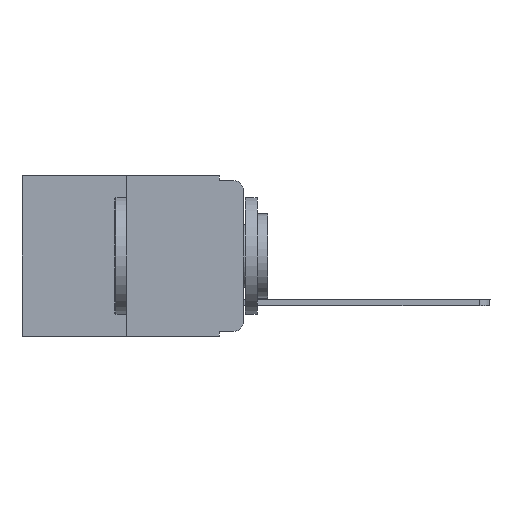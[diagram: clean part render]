
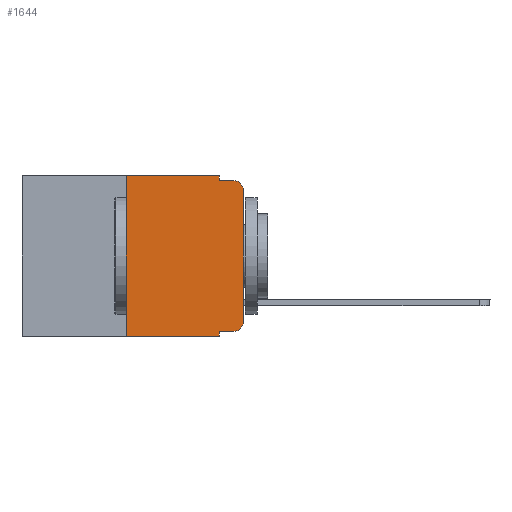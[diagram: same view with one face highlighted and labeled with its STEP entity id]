
A CAD part, left-side view. The second image highlights one B-rep face of the part: STEP entity #1644.
In plain terms, the highlighted planar face has unit normal (-1, 0, 0).
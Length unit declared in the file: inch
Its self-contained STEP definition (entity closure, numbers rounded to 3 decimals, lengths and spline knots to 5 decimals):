
#86 = EDGE_CURVE ( 'NONE', #6465, #8128, #5907, .T. ) ;
#367 = EDGE_CURVE ( 'NONE', #8128, #1295, #6857, .T. ) ;
#413 = DIRECTION ( 'NONE',  ( 0., -1., 0. ) ) ;
#426 = LINE ( 'NONE', #8678, #9998 ) ;
#717 = ORIENTED_EDGE ( 'NONE', *, *, #2191, .T. ) ;
#792 = CARTESIAN_POINT ( 'NONE',  ( 0., 0.051, -0.01 ) ) ;
#1022 = ORIENTED_EDGE ( 'NONE', *, *, #86, .F. ) ;
#1288 = LINE ( 'NONE', #8288, #7747 ) ;
#1295 = VERTEX_POINT ( 'NONE', #792 ) ;
#1339 = LINE ( 'NONE', #3918, #3403 ) ;
#1460 = VECTOR ( 'NONE', #2032, 39.37008 ) ;
#1644 = ADVANCED_FACE ( 'NONE', ( #3389 ), #11293, .F. ) ;
#1742 = CARTESIAN_POINT ( 'NONE',  ( 0., 0.051, 0. ) ) ;
#1980 = AXIS2_PLACEMENT_3D ( 'NONE', #9676, #5297, #2703 ) ;
#2032 = DIRECTION ( 'NONE',  ( 0., 0., 1. ) ) ;
#2186 = VERTEX_POINT ( 'NONE', #10631 ) ;
#2191 = EDGE_CURVE ( 'NONE', #2186, #9659, #3777, .T. ) ;
#2703 = DIRECTION ( 'NONE',  ( 0., 0., -1. ) ) ;
#2757 = ORIENTED_EDGE ( 'NONE', *, *, #10339, .F. ) ;
#2854 = CARTESIAN_POINT ( 'NONE',  ( 0., 0.051, -0.01 ) ) ;
#2925 = DIRECTION ( 'NONE',  ( 0., 0., -1. ) ) ;
#2929 = CARTESIAN_POINT ( 'NONE',  ( 0., 0.02, -0.03 ) ) ;
#3389 = FACE_OUTER_BOUND ( 'NONE', #8650, .T. ) ;
#3397 = VERTEX_POINT ( 'NONE', #9540 ) ;
#3403 = VECTOR ( 'NONE', #4871, 39.37008 ) ;
#3587 = VERTEX_POINT ( 'NONE', #5398 ) ;
#3691 = ORIENTED_EDGE ( 'NONE', *, *, #8465, .T. ) ;
#3777 = LINE ( 'NONE', #9738, #1460 ) ;
#3829 = VECTOR ( 'NONE', #8747, 39.37008 ) ;
#3918 = CARTESIAN_POINT ( 'NONE',  ( 0., 0.051, -0.333 ) ) ;
#4284 = ORIENTED_EDGE ( 'NONE', *, *, #10265, .F. ) ;
#4354 = EDGE_CURVE ( 'NONE', #9659, #6924, #7439, .T. ) ;
#4414 = CARTESIAN_POINT ( 'NONE',  ( 0., 0.051, 0. ) ) ;
#4619 = VECTOR ( 'NONE', #10669, 39.37008 ) ;
#4871 = DIRECTION ( 'NONE',  ( 0., -1., 0. ) ) ;
#5122 = CIRCLE ( 'NONE', #1980, 0.02 ) ;
#5204 = VERTEX_POINT ( 'NONE', #5212 ) ;
#5212 = CARTESIAN_POINT ( 'NONE',  ( 0., 0.02, -0.333 ) ) ;
#5297 = DIRECTION ( 'NONE',  ( -1., 0., 0. ) ) ;
#5398 = CARTESIAN_POINT ( 'NONE',  ( 0., 0.051, -0.333 ) ) ;
#5907 = LINE ( 'NONE', #10479, #3829 ) ;
#6090 = DIRECTION ( 'NONE',  ( 0., 0., 1. ) ) ;
#6147 = AXIS2_PLACEMENT_3D ( 'NONE', #2929, #9511, #9818 ) ;
#6179 = LINE ( 'NONE', #2854, #11106 ) ;
#6301 = CARTESIAN_POINT ( 'NONE',  ( 0., 0.25, 0. ) ) ;
#6394 = EDGE_CURVE ( 'NONE', #3587, #10872, #9156, .T. ) ;
#6465 = VERTEX_POINT ( 'NONE', #6301 ) ;
#6785 = DIRECTION ( 'NONE',  ( 1., 0., 0. ) ) ;
#6857 = LINE ( 'NONE', #1742, #10555 ) ;
#6924 = VERTEX_POINT ( 'NONE', #10465 ) ;
#7076 = CARTESIAN_POINT ( 'NONE',  ( 0., 0.051, -0.343 ) ) ;
#7264 = CARTESIAN_POINT ( 'NONE',  ( 0., 0.051, 0. ) ) ;
#7439 = CIRCLE ( 'NONE', #6147, 0.02 ) ;
#7747 = VECTOR ( 'NONE', #413, 39.37008 ) ;
#8128 = VERTEX_POINT ( 'NONE', #4414 ) ;
#8288 = CARTESIAN_POINT ( 'NONE',  ( 0., 0.473, -0.343 ) ) ;
#8465 = EDGE_CURVE ( 'NONE', #5204, #2186, #5122, .T. ) ;
#8650 = EDGE_LOOP ( 'NONE', ( #717, #11130, #2757, #10474, #1022, #4284, #11305, #9057, #9754, #3691 ) ) ;
#8678 = CARTESIAN_POINT ( 'NONE',  ( 0., 0.25, 0. ) ) ;
#8716 = EDGE_CURVE ( 'NONE', #3397, #10872, #1288, .T. ) ;
#8747 = DIRECTION ( 'NONE',  ( 0., -1., 0. ) ) ;
#8765 = CARTESIAN_POINT ( 'NONE',  ( 0., 0., -0.03 ) ) ;
#8867 = DIRECTION ( 'NONE',  ( 0., -1., 0. ) ) ;
#9057 = ORIENTED_EDGE ( 'NONE', *, *, #6394, .F. ) ;
#9156 = LINE ( 'NONE', #7264, #4619 ) ;
#9511 = DIRECTION ( 'NONE',  ( -1., 0., 0. ) ) ;
#9537 = CARTESIAN_POINT ( 'NONE',  ( 0., 0.473, 0. ) ) ;
#9540 = CARTESIAN_POINT ( 'NONE',  ( 0., 0.25, -0.343 ) ) ;
#9659 = VERTEX_POINT ( 'NONE', #8765 ) ;
#9676 = CARTESIAN_POINT ( 'NONE',  ( 0., 0.02, -0.313 ) ) ;
#9738 = CARTESIAN_POINT ( 'NONE',  ( 0., 0., 0. ) ) ;
#9754 = ORIENTED_EDGE ( 'NONE', *, *, #11072, .T. ) ;
#9818 = DIRECTION ( 'NONE',  ( 0., 0., -1. ) ) ;
#9998 = VECTOR ( 'NONE', #6090, 39.37008 ) ;
#10265 = EDGE_CURVE ( 'NONE', #3397, #6465, #426, .T. ) ;
#10339 = EDGE_CURVE ( 'NONE', #1295, #6924, #6179, .T. ) ;
#10465 = CARTESIAN_POINT ( 'NONE',  ( 0., 0.02, -0.01 ) ) ;
#10474 = ORIENTED_EDGE ( 'NONE', *, *, #367, .F. ) ;
#10479 = CARTESIAN_POINT ( 'NONE',  ( 0., 0.473, 0. ) ) ;
#10555 = VECTOR ( 'NONE', #2925, 39.37008 ) ;
#10605 = AXIS2_PLACEMENT_3D ( 'NONE', #9537, #6785, #10756 ) ;
#10631 = CARTESIAN_POINT ( 'NONE',  ( 0., 0., -0.313 ) ) ;
#10669 = DIRECTION ( 'NONE',  ( 0., 0., -1. ) ) ;
#10756 = DIRECTION ( 'NONE',  ( 0., 0., -1. ) ) ;
#10872 = VERTEX_POINT ( 'NONE', #7076 ) ;
#11072 = EDGE_CURVE ( 'NONE', #3587, #5204, #1339, .T. ) ;
#11106 = VECTOR ( 'NONE', #8867, 39.37008 ) ;
#11130 = ORIENTED_EDGE ( 'NONE', *, *, #4354, .T. ) ;
#11293 = PLANE ( 'NONE',  #10605 ) ;
#11305 = ORIENTED_EDGE ( 'NONE', *, *, #8716, .T. ) ;
